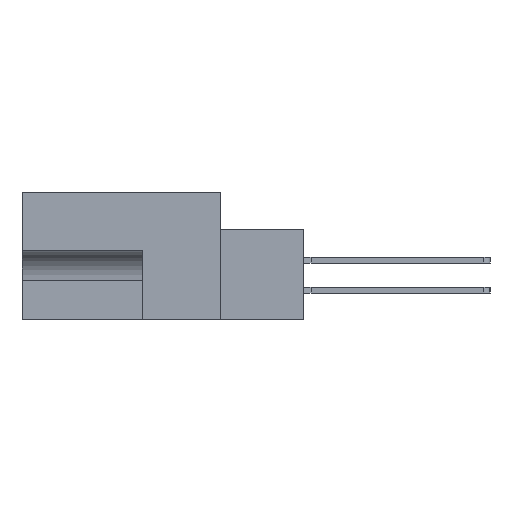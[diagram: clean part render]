
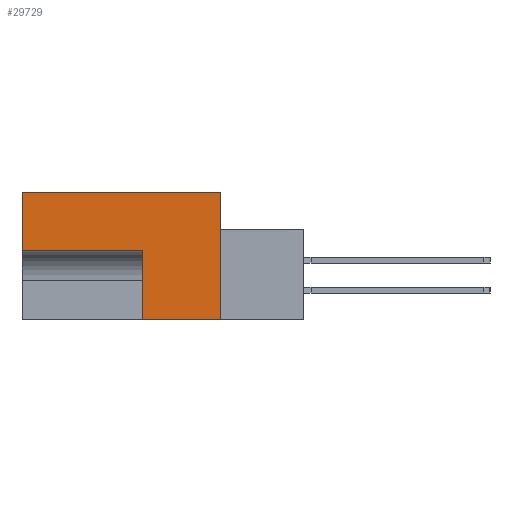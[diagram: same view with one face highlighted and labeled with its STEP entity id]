
A CAD part, left-side view. The second image highlights one B-rep face of the part: STEP entity #29729.
In plain terms, the highlighted planar face has unit normal (-1, 0, 0).
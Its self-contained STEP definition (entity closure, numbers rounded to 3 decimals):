
#1151 = EDGE_CURVE ( 'NONE', #13919, #32745, #4746, .T. ) ;
#1976 = VECTOR ( 'NONE', #37121, 1000. ) ;
#3322 = CARTESIAN_POINT ( 'NONE',  ( 0., 8.255, -13.487 ) ) ;
#4189 = LINE ( 'NONE', #3322, #29807 ) ;
#4746 = LINE ( 'NONE', #39858, #23990 ) ;
#5715 = CARTESIAN_POINT ( 'NONE',  ( 0., 20.955, -6.172 ) ) ;
#7377 = LINE ( 'NONE', #8991, #1976 ) ;
#8621 = DIRECTION ( 'NONE',  ( 0., 1., 0. ) ) ;
#8991 = CARTESIAN_POINT ( 'NONE',  ( 0., -8.814, -13.487 ) ) ;
#10302 = ORIENTED_EDGE ( 'NONE', *, *, #27153, .F. ) ;
#11729 = CARTESIAN_POINT ( 'NONE',  ( 0., 20.955, 0. ) ) ;
#11919 = CARTESIAN_POINT ( 'NONE',  ( 0., 0., 0. ) ) ;
#12355 = ORIENTED_EDGE ( 'NONE', *, *, #38184, .F. ) ;
#13919 = VERTEX_POINT ( 'NONE', #5715 ) ;
#14096 = VERTEX_POINT ( 'NONE', #39026 ) ;
#14694 = LINE ( 'NONE', #21802, #23606 ) ;
#15018 = VERTEX_POINT ( 'NONE', #22793 ) ;
#15475 = FACE_OUTER_BOUND ( 'NONE', #34793, .T. ) ;
#16216 = VECTOR ( 'NONE', #22379, 1000. ) ;
#16253 = DIRECTION ( 'NONE',  ( 0., 0., 1. ) ) ;
#17150 = ORIENTED_EDGE ( 'NONE', *, *, #22319, .F. ) ;
#18062 = DIRECTION ( 'NONE',  ( 0., -1., 0. ) ) ;
#18399 = DIRECTION ( 'NONE',  ( 0., 0., -1. ) ) ;
#19695 = VERTEX_POINT ( 'NONE', #29489 ) ;
#19984 = VERTEX_POINT ( 'NONE', #40484 ) ;
#20680 = EDGE_CURVE ( 'NONE', #19984, #14096, #34968, .T. ) ;
#20918 = CARTESIAN_POINT ( 'NONE',  ( 0., 8.255, -6.172 ) ) ;
#21802 = CARTESIAN_POINT ( 'NONE',  ( 0., 11.506, 0. ) ) ;
#22319 = EDGE_CURVE ( 'NONE', #15018, #13919, #40795, .T. ) ;
#22379 = DIRECTION ( 'NONE',  ( 0., 0., -1. ) ) ;
#22793 = CARTESIAN_POINT ( 'NONE',  ( 0., 8.255, -6.172 ) ) ;
#23493 = EDGE_CURVE ( 'NONE', #19695, #15018, #4189, .T. ) ;
#23606 = VECTOR ( 'NONE', #18062, 1000. ) ;
#23990 = VECTOR ( 'NONE', #33668, 1000. ) ;
#24845 = ORIENTED_EDGE ( 'NONE', *, *, #20680, .F. ) ;
#25756 = AXIS2_PLACEMENT_3D ( 'NONE', #11919, #37160, #18399 ) ;
#26601 = ORIENTED_EDGE ( 'NONE', *, *, #23493, .F. ) ;
#27153 = EDGE_CURVE ( 'NONE', #32745, #19984, #14694, .T. ) ;
#28711 = CARTESIAN_POINT ( 'NONE',  ( 0., 0., 0. ) ) ;
#29489 = CARTESIAN_POINT ( 'NONE',  ( 0., 8.255, -13.487 ) ) ;
#29729 = ADVANCED_FACE ( 'NONE', ( #15475 ), #37307, .F. ) ;
#29807 = VECTOR ( 'NONE', #16253, 1000. ) ;
#31376 = VECTOR ( 'NONE', #8621, 1000. ) ;
#32745 = VERTEX_POINT ( 'NONE', #11729 ) ;
#33668 = DIRECTION ( 'NONE',  ( 0., 0., 1. ) ) ;
#34793 = EDGE_LOOP ( 'NONE', ( #12355, #24845, #10302, #35766, #17150, #26601 ) ) ;
#34968 = LINE ( 'NONE', #28711, #16216 ) ;
#35766 = ORIENTED_EDGE ( 'NONE', *, *, #1151, .F. ) ;
#37121 = DIRECTION ( 'NONE',  ( 0., 1., 0. ) ) ;
#37160 = DIRECTION ( 'NONE',  ( 1., 0., 0. ) ) ;
#37307 = PLANE ( 'NONE',  #25756 ) ;
#38184 = EDGE_CURVE ( 'NONE', #14096, #19695, #7377, .T. ) ;
#39026 = CARTESIAN_POINT ( 'NONE',  ( 0., 0., -13.487 ) ) ;
#39858 = CARTESIAN_POINT ( 'NONE',  ( 0., 20.955, -13.487 ) ) ;
#40484 = CARTESIAN_POINT ( 'NONE',  ( 0., 0., 0. ) ) ;
#40795 = LINE ( 'NONE', #20918, #31376 ) ;
